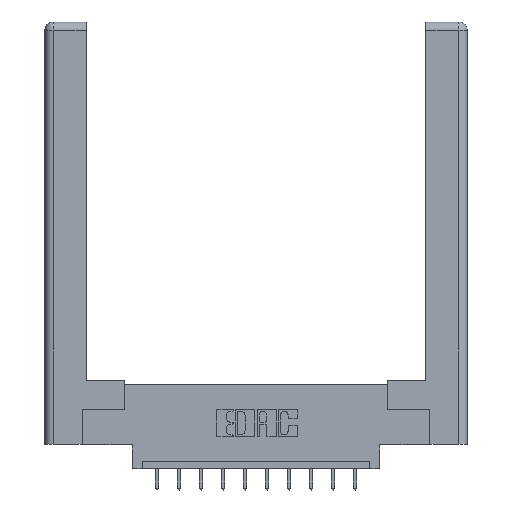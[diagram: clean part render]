
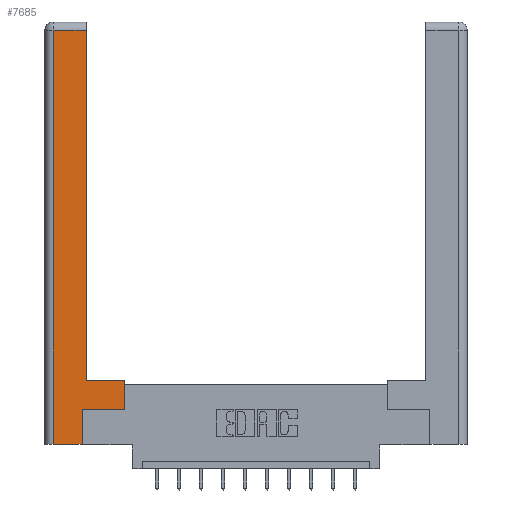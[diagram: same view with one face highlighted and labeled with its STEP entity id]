
A CAD part, top view. The second image highlights one B-rep face of the part: STEP entity #7685.
In plain terms, the highlighted planar face has unit normal (0, 0, 1).
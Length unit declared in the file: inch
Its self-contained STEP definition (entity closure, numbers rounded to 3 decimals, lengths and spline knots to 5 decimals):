
#48 = ORIENTED_EDGE ( 'NONE', *, *, #14168, .T. ) ;
#217 = EDGE_LOOP ( 'NONE', ( #13537, #5775, #694, #12069, #6822, #10064, #48, #3814 ) ) ;
#434 = EDGE_CURVE ( 'NONE', #5616, #2433, #11279, .T. ) ;
#694 = ORIENTED_EDGE ( 'NONE', *, *, #434, .T. ) ;
#1311 = CARTESIAN_POINT ( 'NONE',  ( 0.565, 0.45, 0. ) ) ;
#1630 = EDGE_CURVE ( 'NONE', #4032, #5616, #13817, .T. ) ;
#1799 = LINE ( 'NONE', #6063, #10318 ) ;
#1899 = VECTOR ( 'NONE', #8139, 39.37008 ) ;
#1989 = VERTEX_POINT ( 'NONE', #14013 ) ;
#1998 = CARTESIAN_POINT ( 'NONE',  ( 0., 0., 0. ) ) ;
#2426 = LINE ( 'NONE', #3075, #11674 ) ;
#2433 = VERTEX_POINT ( 'NONE', #9450 ) ;
#2513 = CARTESIAN_POINT ( 'NONE',  ( 0.0615, 0., 0. ) ) ;
#2731 = LINE ( 'NONE', #1311, #4669 ) ;
#3075 = CARTESIAN_POINT ( 'NONE',  ( 0.295, 3., 0. ) ) ;
#3783 = CARTESIAN_POINT ( 'NONE',  ( 0.565, 0.245, 0. ) ) ;
#3814 = ORIENTED_EDGE ( 'NONE', *, *, #7645, .T. ) ;
#4032 = VERTEX_POINT ( 'NONE', #4448 ) ;
#4219 = CARTESIAN_POINT ( 'NONE',  ( 0.265, 0., 0. ) ) ;
#4448 = CARTESIAN_POINT ( 'NONE',  ( 0.295, 2.94, 0. ) ) ;
#4492 = LINE ( 'NONE', #7152, #9875 ) ;
#4669 = VECTOR ( 'NONE', #10206, 39.37008 ) ;
#4886 = CARTESIAN_POINT ( 'NONE',  ( 0.0615, 2.94, 0. ) ) ;
#5520 = VECTOR ( 'NONE', #11340, 39.37008 ) ;
#5616 = VERTEX_POINT ( 'NONE', #11502 ) ;
#5775 = ORIENTED_EDGE ( 'NONE', *, *, #1630, .T. ) ;
#6063 = CARTESIAN_POINT ( 'NONE',  ( 0.265, 0.245, 0. ) ) ;
#6713 = EDGE_CURVE ( 'NONE', #2433, #10469, #4492, .T. ) ;
#6822 = ORIENTED_EDGE ( 'NONE', *, *, #9044, .T. ) ;
#7152 = CARTESIAN_POINT ( 'NONE',  ( 0.265, 0., 0. ) ) ;
#7645 = EDGE_CURVE ( 'NONE', #1989, #13143, #9511, .T. ) ;
#7685 = ADVANCED_FACE ( 'NONE', ( #10717 ), #8679, .F. ) ;
#8139 = DIRECTION ( 'NONE',  ( 1., 0., 0. ) ) ;
#8291 = AXIS2_PLACEMENT_3D ( 'NONE', #1998, #9793, #10966 ) ;
#8679 = PLANE ( 'NONE',  #8291 ) ;
#8773 = DIRECTION ( 'NONE',  ( -1., 0., 0. ) ) ;
#9044 = EDGE_CURVE ( 'NONE', #10469, #11814, #1799, .T. ) ;
#9166 = VECTOR ( 'NONE', #8773, 39.37008 ) ;
#9450 = CARTESIAN_POINT ( 'NONE',  ( 0.0615, 0., 0. ) ) ;
#9511 = LINE ( 'NONE', #13907, #9166 ) ;
#9638 = DIRECTION ( 'NONE',  ( 0., 1., 0. ) ) ;
#9793 = DIRECTION ( 'NONE',  ( 0., 0., -1. ) ) ;
#9875 = VECTOR ( 'NONE', #10670, 39.37008 ) ;
#10064 = ORIENTED_EDGE ( 'NONE', *, *, #13443, .T. ) ;
#10196 = CARTESIAN_POINT ( 'NONE',  ( 0.265, 0.245, 0. ) ) ;
#10206 = DIRECTION ( 'NONE',  ( 0., 1., 0. ) ) ;
#10318 = VECTOR ( 'NONE', #9638, 39.37008 ) ;
#10469 = VERTEX_POINT ( 'NONE', #4219 ) ;
#10565 = CARTESIAN_POINT ( 'NONE',  ( 0.565, 0.245, 0. ) ) ;
#10670 = DIRECTION ( 'NONE',  ( 1., 0., 0. ) ) ;
#10717 = FACE_OUTER_BOUND ( 'NONE', #217, .T. ) ;
#10966 = DIRECTION ( 'NONE',  ( -1., 0., 0. ) ) ;
#10991 = DIRECTION ( 'NONE',  ( 0., 1., 0. ) ) ;
#11279 = LINE ( 'NONE', #2513, #5520 ) ;
#11340 = DIRECTION ( 'NONE',  ( 0., -1., 0. ) ) ;
#11502 = CARTESIAN_POINT ( 'NONE',  ( 0.0615, 2.94, 0. ) ) ;
#11642 = DIRECTION ( 'NONE',  ( -1., 0., 0. ) ) ;
#11674 = VECTOR ( 'NONE', #10991, 39.37008 ) ;
#11814 = VERTEX_POINT ( 'NONE', #10196 ) ;
#12069 = ORIENTED_EDGE ( 'NONE', *, *, #6713, .T. ) ;
#12439 = VECTOR ( 'NONE', #11642, 39.37008 ) ;
#12588 = EDGE_CURVE ( 'NONE', #13143, #4032, #2426, .T. ) ;
#12936 = CARTESIAN_POINT ( 'NONE',  ( 0.295, 0.45, 0. ) ) ;
#13064 = VERTEX_POINT ( 'NONE', #10565 ) ;
#13143 = VERTEX_POINT ( 'NONE', #12936 ) ;
#13443 = EDGE_CURVE ( 'NONE', #11814, #13064, #13900, .T. ) ;
#13537 = ORIENTED_EDGE ( 'NONE', *, *, #12588, .T. ) ;
#13817 = LINE ( 'NONE', #4886, #12439 ) ;
#13900 = LINE ( 'NONE', #3783, #1899 ) ;
#13907 = CARTESIAN_POINT ( 'NONE',  ( 0.295, 0.45, 0. ) ) ;
#14013 = CARTESIAN_POINT ( 'NONE',  ( 0.565, 0.45, 0. ) ) ;
#14168 = EDGE_CURVE ( 'NONE', #13064, #1989, #2731, .T. ) ;
